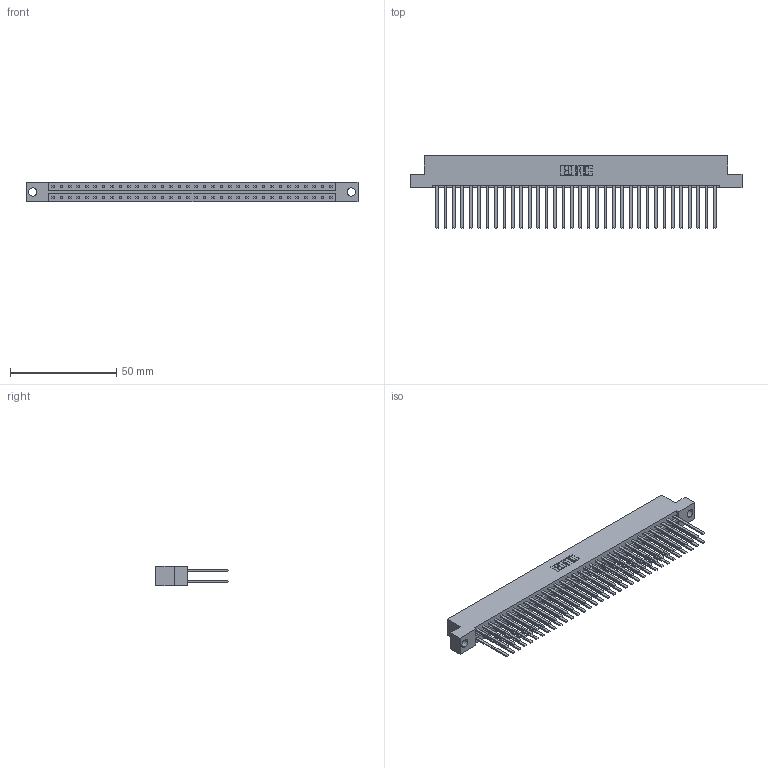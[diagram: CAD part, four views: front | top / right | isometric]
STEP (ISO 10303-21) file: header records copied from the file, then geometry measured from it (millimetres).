
FILE_DESCRIPTION (( 'STEP AP203' ), '1' );
FILE_NAME ('333-068-544-204.STEP', '2018-08-04T13:18:34', ( '' ), ( '' ), 'SwSTEP 2.0', 'SolidWorks 2016', '' );
FILE_SCHEMA (( 'CONFIG_CONTROL_DESIGN' ));
Length unit declared in the file: inch
Products named in the file (3): 333 Part_Flush - .156 Dia - TH; 345-292-001_345-293-144; 333-068-544-204
Assembly tree (69 placements, depth 2):
  333-068-544-204
    333 Part_Flush - .156 Dia - TH
    345-292-001_345-293-144  x68
Bounding box: 156.26 x 34.3 x 9.4 mm (x, y, z)
Volume: 16743.9 mm3; surface area: 22578.1 mm2
Topology: 69 solids, 69 shells, 3242 faces, 9627 edges, 6326 vertices
Faces by surface type: plane 2246, cylinder 996
Entity records: 22727 total; most frequent: CARTESIAN_POINT 3774, ORIENTED_EDGE 3710, DIRECTION 3235, EDGE_CURVE 1855, VECTOR 1731, LINE 1731, VERTEX_POINT 1234, AXIS2_PLACEMENT_3D 752
